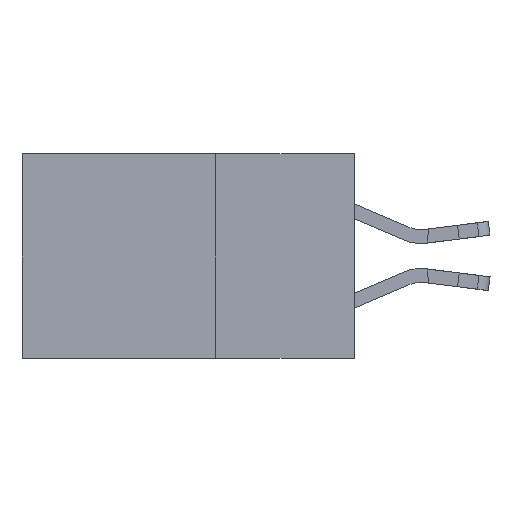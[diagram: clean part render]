
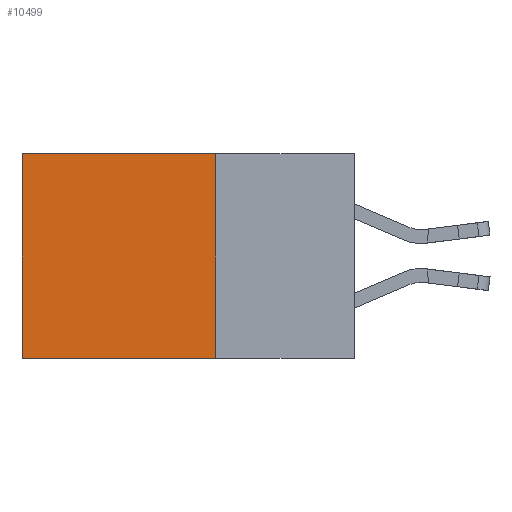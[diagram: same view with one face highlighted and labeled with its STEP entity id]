
A CAD part, left-side view. The second image highlights one B-rep face of the part: STEP entity #10499.
In plain terms, the highlighted planar face has unit normal (-1, 0, 0).
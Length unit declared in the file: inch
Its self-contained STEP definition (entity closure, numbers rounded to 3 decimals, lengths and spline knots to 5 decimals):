
#796 = AXIS2_PLACEMENT_3D ( 'NONE', #10302, #13033, #4894 ) ;
#1295 = VERTEX_POINT ( 'NONE', #2872 ) ;
#1361 = EDGE_CURVE ( 'NONE', #12225, #9627, #6645, .T. ) ;
#2468 = EDGE_CURVE ( 'NONE', #9627, #1295, #6391, .T. ) ;
#2872 = CARTESIAN_POINT ( 'NONE',  ( 0.2615, 0.6, -0.37 ) ) ;
#2990 = LINE ( 'NONE', #9930, #9766 ) ;
#3443 = ORIENTED_EDGE ( 'NONE', *, *, #5471, .F. ) ;
#4128 = VECTOR ( 'NONE', #7978, 39.37008 ) ;
#4894 = DIRECTION ( 'NONE',  ( 0., 0., -1. ) ) ;
#5471 = EDGE_CURVE ( 'NONE', #12225, #14189, #11345, .T. ) ;
#6391 = LINE ( 'NONE', #17412, #16777 ) ;
#6525 = ORIENTED_EDGE ( 'NONE', *, *, #1361, .T. ) ;
#6645 = LINE ( 'NONE', #8461, #9378 ) ;
#7624 = EDGE_CURVE ( 'NONE', #14189, #1295, #2990, .T. ) ;
#7720 = EDGE_LOOP ( 'NONE', ( #11422, #16917, #3443, #6525 ) ) ;
#7978 = DIRECTION ( 'NONE',  ( 0., 0., -1. ) ) ;
#8461 = CARTESIAN_POINT ( 'NONE',  ( 0.2615, 0.25, 0. ) ) ;
#8502 = DIRECTION ( 'NONE',  ( 0., 1., 0. ) ) ;
#9103 = CARTESIAN_POINT ( 'NONE',  ( 0.2615, 0.25, -0.37 ) ) ;
#9205 = CARTESIAN_POINT ( 'NONE',  ( 0.2615, 0.25, 0. ) ) ;
#9378 = VECTOR ( 'NONE', #8502, 39.37008 ) ;
#9627 = VERTEX_POINT ( 'NONE', #9838 ) ;
#9766 = VECTOR ( 'NONE', #9879, 39.37008 ) ;
#9838 = CARTESIAN_POINT ( 'NONE',  ( 0.2615, 0.6, 0. ) ) ;
#9879 = DIRECTION ( 'NONE',  ( 0., 1., 0. ) ) ;
#9930 = CARTESIAN_POINT ( 'NONE',  ( 0.2615, 0.25, -0.37 ) ) ;
#10290 = CARTESIAN_POINT ( 'NONE',  ( 0.2615, 0.25, -0.37 ) ) ;
#10302 = CARTESIAN_POINT ( 'NONE',  ( 0.2615, 0.25, -0.37 ) ) ;
#10499 = ADVANCED_FACE ( 'NONE', ( #17309 ), #15655, .F. ) ;
#11345 = LINE ( 'NONE', #9103, #4128 ) ;
#11422 = ORIENTED_EDGE ( 'NONE', *, *, #2468, .T. ) ;
#12225 = VERTEX_POINT ( 'NONE', #9205 ) ;
#13033 = DIRECTION ( 'NONE',  ( 1., 0., 0. ) ) ;
#14189 = VERTEX_POINT ( 'NONE', #10290 ) ;
#15655 = PLANE ( 'NONE',  #796 ) ;
#16777 = VECTOR ( 'NONE', #17389, 39.37008 ) ;
#16917 = ORIENTED_EDGE ( 'NONE', *, *, #7624, .F. ) ;
#17309 = FACE_OUTER_BOUND ( 'NONE', #7720, .T. ) ;
#17389 = DIRECTION ( 'NONE',  ( 0., 0., -1. ) ) ;
#17412 = CARTESIAN_POINT ( 'NONE',  ( 0.2615, 0.6, -0.37 ) ) ;
